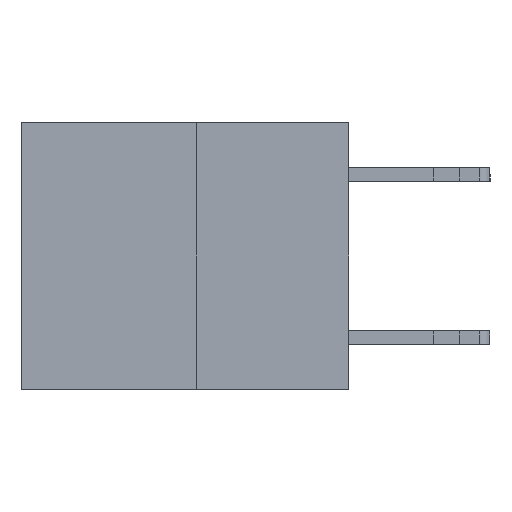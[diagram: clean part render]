
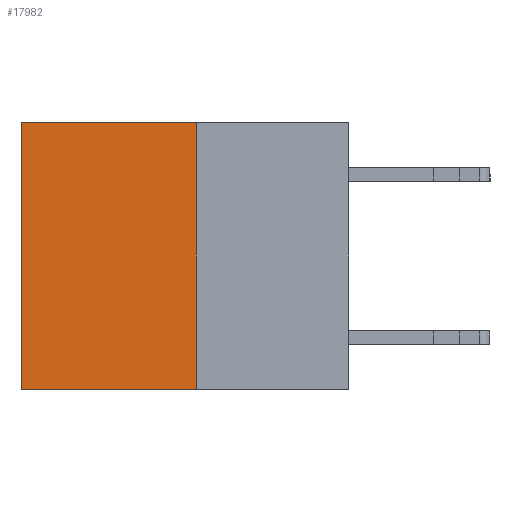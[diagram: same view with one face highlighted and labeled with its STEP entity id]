
A CAD part, left-side view. The second image highlights one B-rep face of the part: STEP entity #17982.
In plain terms, the highlighted planar face has unit normal (-1, 0, 0).
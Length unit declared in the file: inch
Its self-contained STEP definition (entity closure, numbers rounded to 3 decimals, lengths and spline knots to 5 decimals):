
#117 = EDGE_CURVE ( 'NONE', #7229, #14813, #16753, .T. ) ;
#419 = DIRECTION ( 'NONE',  ( 0., 1., 0. ) ) ;
#2542 = DIRECTION ( 'NONE',  ( 0., 0., -1. ) ) ;
#2893 = DIRECTION ( 'NONE',  ( 1., 0., 0. ) ) ;
#3523 = DIRECTION ( 'NONE',  ( 0., 0., -1. ) ) ;
#3614 = CARTESIAN_POINT ( 'NONE',  ( 0.3165, 0.28, -0.49 ) ) ;
#4177 = PLANE ( 'NONE',  #11921 ) ;
#4591 = CARTESIAN_POINT ( 'NONE',  ( 0.3165, 0.28, -0.49 ) ) ;
#4683 = VECTOR ( 'NONE', #5083, 39.37008 ) ;
#5083 = DIRECTION ( 'NONE',  ( 0., 1., 0. ) ) ;
#6054 = VECTOR ( 'NONE', #3523, 39.37008 ) ;
#6265 = DIRECTION ( 'NONE',  ( 0., 0., -1. ) ) ;
#6526 = ORIENTED_EDGE ( 'NONE', *, *, #9948, .T. ) ;
#6626 = EDGE_CURVE ( 'NONE', #13906, #12128, #13348, .T. ) ;
#6675 = CARTESIAN_POINT ( 'NONE',  ( 0.3165, 0.28, 0. ) ) ;
#6898 = VECTOR ( 'NONE', #2542, 39.37008 ) ;
#7098 = VECTOR ( 'NONE', #419, 39.37008 ) ;
#7229 = VERTEX_POINT ( 'NONE', #9354 ) ;
#8202 = CARTESIAN_POINT ( 'NONE',  ( 0.3165, 0.28, -0.49 ) ) ;
#8491 = ORIENTED_EDGE ( 'NONE', *, *, #17672, .F. ) ;
#9354 = CARTESIAN_POINT ( 'NONE',  ( 0.3165, 0.6, 0. ) ) ;
#9948 = EDGE_CURVE ( 'NONE', #13906, #7229, #19697, .T. ) ;
#10470 = LINE ( 'NONE', #3614, #4683 ) ;
#10514 = CARTESIAN_POINT ( 'NONE',  ( 0.3165, 0.6, -0.49 ) ) ;
#11921 = AXIS2_PLACEMENT_3D ( 'NONE', #4591, #2893, #6265 ) ;
#12128 = VERTEX_POINT ( 'NONE', #13264 ) ;
#12755 = FACE_OUTER_BOUND ( 'NONE', #15588, .T. ) ;
#13264 = CARTESIAN_POINT ( 'NONE',  ( 0.3165, 0.28, -0.49 ) ) ;
#13348 = LINE ( 'NONE', #8202, #6054 ) ;
#13444 = CARTESIAN_POINT ( 'NONE',  ( 0.3165, 0.6, -0.49 ) ) ;
#13906 = VERTEX_POINT ( 'NONE', #6675 ) ;
#14813 = VERTEX_POINT ( 'NONE', #13444 ) ;
#15588 = EDGE_LOOP ( 'NONE', ( #17295, #8491, #19483, #6526 ) ) ;
#16753 = LINE ( 'NONE', #10514, #6898 ) ;
#17295 = ORIENTED_EDGE ( 'NONE', *, *, #117, .T. ) ;
#17672 = EDGE_CURVE ( 'NONE', #12128, #14813, #10470, .T. ) ;
#17982 = ADVANCED_FACE ( 'NONE', ( #12755 ), #4177, .F. ) ;
#18065 = CARTESIAN_POINT ( 'NONE',  ( 0.3165, 0.28, 0. ) ) ;
#19483 = ORIENTED_EDGE ( 'NONE', *, *, #6626, .F. ) ;
#19697 = LINE ( 'NONE', #18065, #7098 ) ;
